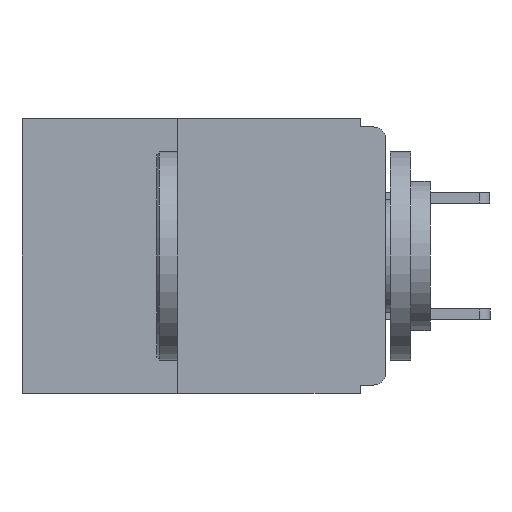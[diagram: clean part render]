
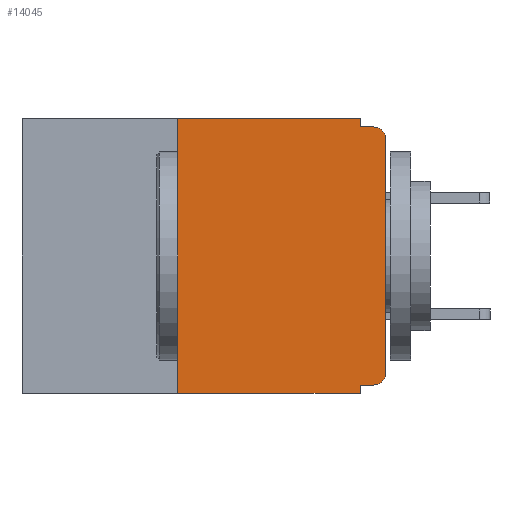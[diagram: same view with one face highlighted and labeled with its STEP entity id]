
A CAD part, left-side view. The second image highlights one B-rep face of the part: STEP entity #14045.
In plain terms, the highlighted planar face has unit normal (-1, 0, 0).
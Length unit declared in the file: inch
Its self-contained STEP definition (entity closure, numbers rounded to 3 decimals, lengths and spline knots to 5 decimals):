
#92 = VERTEX_POINT ( 'NONE', #19441 ) ;
#478 = EDGE_CURVE ( 'NONE', #22188, #92, #24880, .T. ) ;
#913 = ORIENTED_EDGE ( 'NONE', *, *, #12023, .F. ) ;
#965 = VERTEX_POINT ( 'NONE', #25592 ) ;
#1081 = VECTOR ( 'NONE', #17149, 39.37008 ) ;
#1108 = VERTEX_POINT ( 'NONE', #21665 ) ;
#1238 = EDGE_CURVE ( 'NONE', #18837, #25590, #21039, .T. ) ;
#1772 = ORIENTED_EDGE ( 'NONE', *, *, #1238, .F. ) ;
#1875 = ORIENTED_EDGE ( 'NONE', *, *, #21607, .T. ) ;
#1924 = PLANE ( 'NONE',  #4348 ) ;
#1928 = VECTOR ( 'NONE', #16466, 39.37008 ) ;
#1962 = VERTEX_POINT ( 'NONE', #22817 ) ;
#2113 = VERTEX_POINT ( 'NONE', #5489 ) ;
#2137 = FACE_OUTER_BOUND ( 'NONE', #26330, .T. ) ;
#2225 = LINE ( 'NONE', #11665, #12935 ) ;
#2290 = CARTESIAN_POINT ( 'NONE',  ( 0., 0.25, -0.33 ) ) ;
#2630 = VECTOR ( 'NONE', #2796, 39.37008 ) ;
#2796 = DIRECTION ( 'NONE',  ( 0., -1., 0. ) ) ;
#3197 = DIRECTION ( 'NONE',  ( -1., 0., 0. ) ) ;
#3466 = CARTESIAN_POINT ( 'NONE',  ( 0., 0.25, 0. ) ) ;
#3880 = CARTESIAN_POINT ( 'NONE',  ( 0., 0.437, -0.33 ) ) ;
#4171 = DIRECTION ( 'NONE',  ( 0., 0., -1. ) ) ;
#4348 = AXIS2_PLACEMENT_3D ( 'NONE', #8356, #16829, #4171 ) ;
#5035 = DIRECTION ( 'NONE',  ( 0., -1., 0. ) ) ;
#5489 = CARTESIAN_POINT ( 'NONE',  ( 0., 0.015, -0.01 ) ) ;
#6823 = CARTESIAN_POINT ( 'NONE',  ( 0., 0.031, -0.01 ) ) ;
#7457 = CARTESIAN_POINT ( 'NONE',  ( 0., 0.437, 0. ) ) ;
#8356 = CARTESIAN_POINT ( 'NONE',  ( 0., 0.437, 0. ) ) ;
#9014 = LINE ( 'NONE', #23793, #24874 ) ;
#10269 = CARTESIAN_POINT ( 'NONE',  ( 0., 0.031, 0. ) ) ;
#10613 = CARTESIAN_POINT ( 'NONE',  ( 0., 0.25, -0.33 ) ) ;
#10892 = ORIENTED_EDGE ( 'NONE', *, *, #25653, .T. ) ;
#11337 = EDGE_CURVE ( 'NONE', #24368, #2113, #9014, .T. ) ;
#11564 = ORIENTED_EDGE ( 'NONE', *, *, #14826, .F. ) ;
#11665 = CARTESIAN_POINT ( 'NONE',  ( 0., 0.031, -0.33 ) ) ;
#11926 = DIRECTION ( 'NONE',  ( -1., 0., 0. ) ) ;
#12023 = EDGE_CURVE ( 'NONE', #25590, #1108, #2225, .T. ) ;
#12262 = CARTESIAN_POINT ( 'NONE',  ( 0., 0., 0. ) ) ;
#12269 = CARTESIAN_POINT ( 'NONE',  ( 0., 0.015, -0.32 ) ) ;
#12935 = VECTOR ( 'NONE', #19968, 39.37008 ) ;
#13239 = VECTOR ( 'NONE', #18653, 39.37008 ) ;
#13432 = EDGE_CURVE ( 'NONE', #24256, #1108, #22921, .T. ) ;
#14045 = ADVANCED_FACE ( 'NONE', ( #2137 ), #1924, .F. ) ;
#14299 = CIRCLE ( 'NONE', #26322, 0.015 ) ;
#14826 = EDGE_CURVE ( 'NONE', #24256, #22188, #21585, .T. ) ;
#15267 = AXIS2_PLACEMENT_3D ( 'NONE', #15887, #3197, #18008 ) ;
#15732 = ORIENTED_EDGE ( 'NONE', *, *, #13432, .T. ) ;
#15887 = CARTESIAN_POINT ( 'NONE',  ( 0., 0.015, -0.305 ) ) ;
#16466 = DIRECTION ( 'NONE',  ( 0., 0., 1. ) ) ;
#16529 = DIRECTION ( 'NONE',  ( 0., 0., -1. ) ) ;
#16690 = CIRCLE ( 'NONE', #15267, 0.015 ) ;
#16829 = DIRECTION ( 'NONE',  ( 1., 0., 0. ) ) ;
#16951 = EDGE_CURVE ( 'NONE', #965, #1962, #24273, .T. ) ;
#17149 = DIRECTION ( 'NONE',  ( 0., 0., 1. ) ) ;
#17208 = VECTOR ( 'NONE', #16529, 39.37008 ) ;
#17648 = EDGE_CURVE ( 'NONE', #92, #24368, #17883, .T. ) ;
#17883 = LINE ( 'NONE', #10269, #17208 ) ;
#18008 = DIRECTION ( 'NONE',  ( 0., 0., -1. ) ) ;
#18447 = ORIENTED_EDGE ( 'NONE', *, *, #11337, .F. ) ;
#18653 = DIRECTION ( 'NONE',  ( 0., -1., 0. ) ) ;
#18837 = VERTEX_POINT ( 'NONE', #12269 ) ;
#19441 = CARTESIAN_POINT ( 'NONE',  ( 0., 0.031, 0. ) ) ;
#19962 = CARTESIAN_POINT ( 'NONE',  ( 0., 0.031, -0.32 ) ) ;
#19968 = DIRECTION ( 'NONE',  ( 0., 0., -1. ) ) ;
#20447 = ORIENTED_EDGE ( 'NONE', *, *, #17648, .F. ) ;
#21039 = LINE ( 'NONE', #26055, #26397 ) ;
#21585 = LINE ( 'NONE', #2290, #1081 ) ;
#21607 = EDGE_CURVE ( 'NONE', #18837, #965, #16690, .T. ) ;
#21665 = CARTESIAN_POINT ( 'NONE',  ( 0., 0.031, -0.33 ) ) ;
#22188 = VERTEX_POINT ( 'NONE', #3466 ) ;
#22817 = CARTESIAN_POINT ( 'NONE',  ( 0., 0., -0.025 ) ) ;
#22896 = ORIENTED_EDGE ( 'NONE', *, *, #478, .F. ) ;
#22921 = LINE ( 'NONE', #3880, #13239 ) ;
#23766 = DIRECTION ( 'NONE',  ( 0., 1., 0. ) ) ;
#23793 = CARTESIAN_POINT ( 'NONE',  ( 0., 0., -0.01 ) ) ;
#24244 = ORIENTED_EDGE ( 'NONE', *, *, #16951, .T. ) ;
#24256 = VERTEX_POINT ( 'NONE', #10613 ) ;
#24273 = LINE ( 'NONE', #12262, #1928 ) ;
#24279 = CARTESIAN_POINT ( 'NONE',  ( 0., 0.015, -0.025 ) ) ;
#24368 = VERTEX_POINT ( 'NONE', #6823 ) ;
#24874 = VECTOR ( 'NONE', #5035, 39.37008 ) ;
#24880 = LINE ( 'NONE', #7457, #2630 ) ;
#25590 = VERTEX_POINT ( 'NONE', #19962 ) ;
#25592 = CARTESIAN_POINT ( 'NONE',  ( 0., 0., -0.305 ) ) ;
#25653 = EDGE_CURVE ( 'NONE', #1962, #2113, #14299, .T. ) ;
#26055 = CARTESIAN_POINT ( 'NONE',  ( 0., 0., -0.32 ) ) ;
#26305 = DIRECTION ( 'NONE',  ( 0., 0., -1. ) ) ;
#26322 = AXIS2_PLACEMENT_3D ( 'NONE', #24279, #11926, #26305 ) ;
#26330 = EDGE_LOOP ( 'NONE', ( #24244, #10892, #18447, #20447, #22896, #11564, #15732, #913, #1772, #1875 ) ) ;
#26397 = VECTOR ( 'NONE', #23766, 39.37008 ) ;
